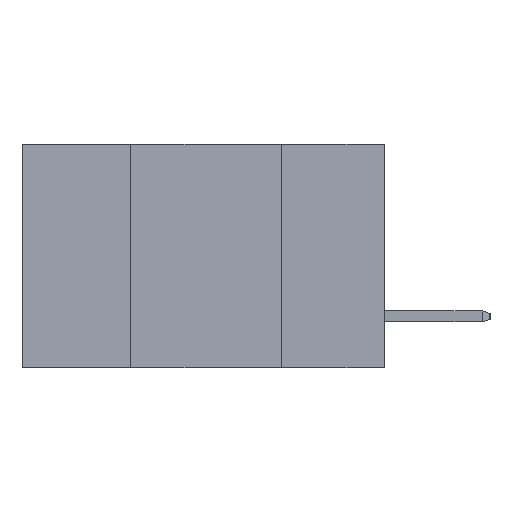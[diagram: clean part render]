
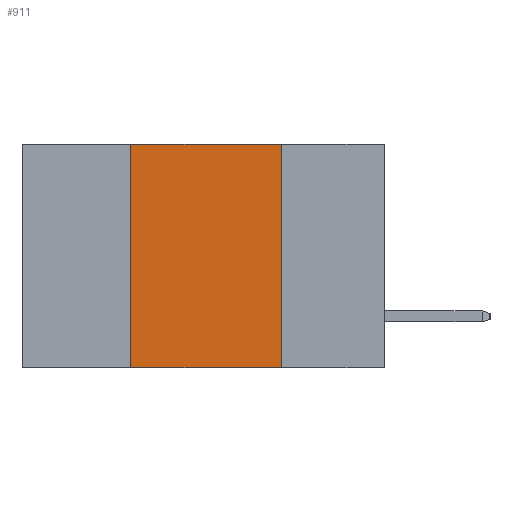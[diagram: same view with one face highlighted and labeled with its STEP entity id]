
A CAD part, left-side view. The second image highlights one B-rep face of the part: STEP entity #911.
In plain terms, the highlighted planar face has unit normal (-1, 0, 0).
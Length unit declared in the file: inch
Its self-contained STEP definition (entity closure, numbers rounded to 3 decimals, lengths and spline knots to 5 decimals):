
#368 = VERTEX_POINT ( 'NONE', #9909 ) ;
#377 = LINE ( 'NONE', #2770, #13782 ) ;
#408 = CARTESIAN_POINT ( 'NONE',  ( 0., 0.42, 0. ) ) ;
#911 = ADVANCED_FACE ( 'NONE', ( #9095 ), #3172, .F. ) ;
#1447 = EDGE_CURVE ( 'NONE', #5616, #9604, #8291, .T. ) ;
#1690 = CARTESIAN_POINT ( 'NONE',  ( 0., 0.42, 0. ) ) ;
#2522 = AXIS2_PLACEMENT_3D ( 'NONE', #9383, #16274, #10761 ) ;
#2770 = CARTESIAN_POINT ( 'NONE',  ( 0., 0.6, -0.37 ) ) ;
#3085 = DIRECTION ( 'NONE',  ( 0., -1., 0. ) ) ;
#3106 = LINE ( 'NONE', #8243, #3521 ) ;
#3172 = PLANE ( 'NONE',  #2522 ) ;
#3519 = CARTESIAN_POINT ( 'NONE',  ( 0., 0.17, 0. ) ) ;
#3521 = VECTOR ( 'NONE', #15794, 39.37008 ) ;
#3585 = EDGE_CURVE ( 'NONE', #5616, #368, #377, .T. ) ;
#3658 = ORIENTED_EDGE ( 'NONE', *, *, #1447, .F. ) ;
#4401 = CARTESIAN_POINT ( 'NONE',  ( 0., 0.17, 0. ) ) ;
#4768 = EDGE_CURVE ( 'NONE', #5827, #368, #16582, .T. ) ;
#5616 = VERTEX_POINT ( 'NONE', #8085 ) ;
#5827 = VERTEX_POINT ( 'NONE', #4401 ) ;
#6483 = VECTOR ( 'NONE', #7530, 39.37008 ) ;
#7530 = DIRECTION ( 'NONE',  ( 0., 0., -1. ) ) ;
#7887 = VECTOR ( 'NONE', #9440, 39.37008 ) ;
#7970 = EDGE_CURVE ( 'NONE', #9604, #5827, #3106, .T. ) ;
#8085 = CARTESIAN_POINT ( 'NONE',  ( 0., 0.42, -0.37 ) ) ;
#8243 = CARTESIAN_POINT ( 'NONE',  ( 0., 0.6, 0. ) ) ;
#8291 = LINE ( 'NONE', #1690, #7887 ) ;
#9095 = FACE_OUTER_BOUND ( 'NONE', #9264, .T. ) ;
#9264 = EDGE_LOOP ( 'NONE', ( #13085, #16051, #3658, #10080 ) ) ;
#9383 = CARTESIAN_POINT ( 'NONE',  ( 0., 0.6, 0. ) ) ;
#9440 = DIRECTION ( 'NONE',  ( 0., 0., 1. ) ) ;
#9604 = VERTEX_POINT ( 'NONE', #408 ) ;
#9909 = CARTESIAN_POINT ( 'NONE',  ( 0., 0.17, -0.37 ) ) ;
#10080 = ORIENTED_EDGE ( 'NONE', *, *, #3585, .T. ) ;
#10761 = DIRECTION ( 'NONE',  ( 0., 0., -1. ) ) ;
#13085 = ORIENTED_EDGE ( 'NONE', *, *, #4768, .F. ) ;
#13782 = VECTOR ( 'NONE', #3085, 39.37008 ) ;
#15794 = DIRECTION ( 'NONE',  ( 0., -1., 0. ) ) ;
#16051 = ORIENTED_EDGE ( 'NONE', *, *, #7970, .F. ) ;
#16274 = DIRECTION ( 'NONE',  ( 1., 0., 0. ) ) ;
#16582 = LINE ( 'NONE', #3519, #6483 ) ;
